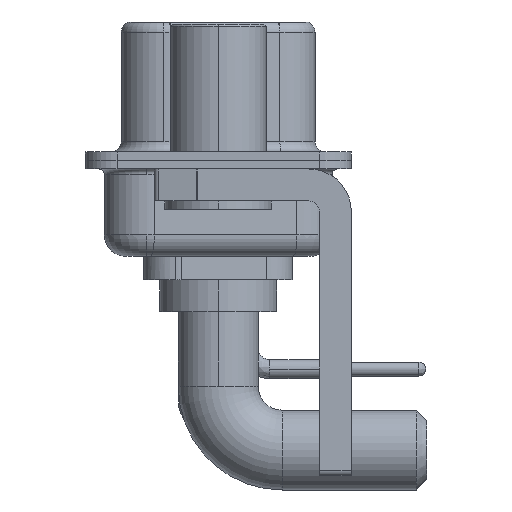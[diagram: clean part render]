
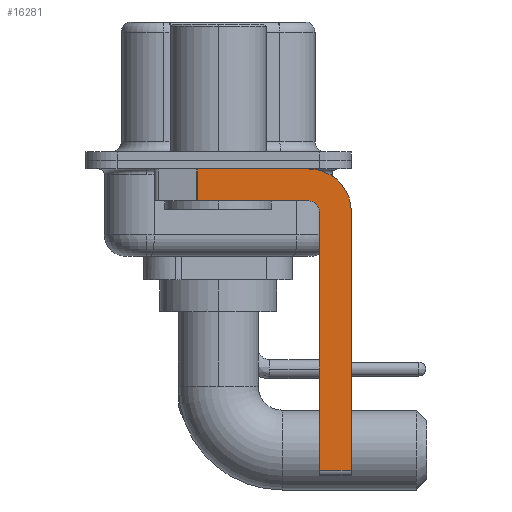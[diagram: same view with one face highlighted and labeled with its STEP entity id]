
A CAD part, left-side view. The second image highlights one B-rep face of the part: STEP entity #16281.
In plain terms, the highlighted planar face has unit normal (-1, 0, 0).
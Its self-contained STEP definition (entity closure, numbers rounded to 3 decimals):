
#114 = CARTESIAN_POINT ( 'NONE',  ( -2.9, -4.75, -14.55 ) ) ;
#766 = PLANE ( 'NONE',  #11342 ) ;
#829 = AXIS2_PLACEMENT_3D ( 'NONE', #30278, #24934, #20228 ) ;
#917 = DIRECTION ( 'NONE',  ( 0., 0., -1. ) ) ;
#1268 = VERTEX_POINT ( 'NONE', #13656 ) ;
#1734 = EDGE_CURVE ( 'NONE', #8570, #30582, #24384, .T. ) ;
#3260 = DIRECTION ( 'NONE',  ( 1., 0., 0. ) ) ;
#5506 = LINE ( 'NONE', #14772, #15397 ) ;
#5513 = EDGE_CURVE ( 'NONE', #26261, #11676, #11392, .T. ) ;
#5656 = CARTESIAN_POINT ( 'NONE',  ( -2.9, -4.75, -2.4 ) ) ;
#6050 = CARTESIAN_POINT ( 'NONE',  ( -2.9, -4.25, -2.4 ) ) ;
#6132 = EDGE_LOOP ( 'NONE', ( #12353, #15788, #12159, #10398, #16314, #27334, #27107, #17771 ) ) ;
#6307 = DIRECTION ( 'NONE',  ( 0., 0., -1. ) ) ;
#7165 = DIRECTION ( 'NONE',  ( 0., -1., 0. ) ) ;
#8091 = DIRECTION ( 'NONE',  ( 1., 0., 0. ) ) ;
#8570 = VERTEX_POINT ( 'NONE', #5656 ) ;
#8659 = CARTESIAN_POINT ( 'NONE',  ( -2.9, 0.978, -1.9 ) ) ;
#10398 = ORIENTED_EDGE ( 'NONE', *, *, #1734, .F. ) ;
#10768 = CARTESIAN_POINT ( 'NONE',  ( -2.9, 0.978, -0.4 ) ) ;
#11250 = EDGE_CURVE ( 'NONE', #11676, #1268, #25630, .T. ) ;
#11342 = AXIS2_PLACEMENT_3D ( 'NONE', #15207, #3260, #917 ) ;
#11392 = LINE ( 'NONE', #13289, #28245 ) ;
#11676 = VERTEX_POINT ( 'NONE', #26122 ) ;
#12008 = VERTEX_POINT ( 'NONE', #12074 ) ;
#12074 = CARTESIAN_POINT ( 'NONE',  ( -2.9, 0.978, -1.9 ) ) ;
#12159 = ORIENTED_EDGE ( 'NONE', *, *, #21912, .F. ) ;
#12353 = ORIENTED_EDGE ( 'NONE', *, *, #5513, .F. ) ;
#12470 = VERTEX_POINT ( 'NONE', #114 ) ;
#12634 = LINE ( 'NONE', #24431, #13814 ) ;
#13289 = CARTESIAN_POINT ( 'NONE',  ( -2.9, 3., -0.4 ) ) ;
#13373 = VERTEX_POINT ( 'NONE', #30831 ) ;
#13656 = CARTESIAN_POINT ( 'NONE',  ( -2.9, -6.25, -2.4 ) ) ;
#13814 = VECTOR ( 'NONE', #7165, 1000. ) ;
#14609 = AXIS2_PLACEMENT_3D ( 'NONE', #6050, #8091, #17840 ) ;
#14772 = CARTESIAN_POINT ( 'NONE',  ( -2.9, -4.75, -14.8 ) ) ;
#15166 = CARTESIAN_POINT ( 'NONE',  ( -2.9, -4.25, -1.9 ) ) ;
#15207 = CARTESIAN_POINT ( 'NONE',  ( -2.9, -4.25, -2.4 ) ) ;
#15327 = EDGE_CURVE ( 'NONE', #12470, #13373, #12634, .T. ) ;
#15397 = VECTOR ( 'NONE', #29210, 1000. ) ;
#15788 = ORIENTED_EDGE ( 'NONE', *, *, #19373, .T. ) ;
#16205 = VECTOR ( 'NONE', #29453, 1000. ) ;
#16281 = ADVANCED_FACE ( 'NONE', ( #22269 ), #766, .F. ) ;
#16314 = ORIENTED_EDGE ( 'NONE', *, *, #18359, .F. ) ;
#17002 = CARTESIAN_POINT ( 'NONE',  ( -2.9, -6.25, -2.4 ) ) ;
#17771 = ORIENTED_EDGE ( 'NONE', *, *, #11250, .F. ) ;
#17840 = DIRECTION ( 'NONE',  ( 0., 0., -1. ) ) ;
#18359 = EDGE_CURVE ( 'NONE', #12470, #8570, #5506, .T. ) ;
#18731 = LINE ( 'NONE', #17002, #25343 ) ;
#19373 = EDGE_CURVE ( 'NONE', #26261, #12008, #27505, .T. ) ;
#20228 = DIRECTION ( 'NONE',  ( 0., 0., 1. ) ) ;
#20984 = DIRECTION ( 'NONE',  ( 0., -1., 0. ) ) ;
#21912 = EDGE_CURVE ( 'NONE', #30582, #12008, #24580, .T. ) ;
#22269 = FACE_OUTER_BOUND ( 'NONE', #6132, .T. ) ;
#23938 = EDGE_CURVE ( 'NONE', #1268, #13373, #18731, .T. ) ;
#24297 = CARTESIAN_POINT ( 'NONE',  ( -2.9, -4.25, -1.9 ) ) ;
#24384 = CIRCLE ( 'NONE', #829, 0.5 ) ;
#24431 = CARTESIAN_POINT ( 'NONE',  ( -2.9, -4.25, -14.55 ) ) ;
#24468 = VECTOR ( 'NONE', #6307, 1000. ) ;
#24580 = LINE ( 'NONE', #15166, #16205 ) ;
#24934 = DIRECTION ( 'NONE',  ( -1., 0., 0. ) ) ;
#25343 = VECTOR ( 'NONE', #26259, 1000. ) ;
#25630 = CIRCLE ( 'NONE', #14609, 2. ) ;
#26122 = CARTESIAN_POINT ( 'NONE',  ( -2.9, -4.25, -0.4 ) ) ;
#26259 = DIRECTION ( 'NONE',  ( 0., 0., -1. ) ) ;
#26261 = VERTEX_POINT ( 'NONE', #10768 ) ;
#27107 = ORIENTED_EDGE ( 'NONE', *, *, #23938, .F. ) ;
#27334 = ORIENTED_EDGE ( 'NONE', *, *, #15327, .T. ) ;
#27505 = LINE ( 'NONE', #8659, #24468 ) ;
#28245 = VECTOR ( 'NONE', #20984, 1000. ) ;
#29210 = DIRECTION ( 'NONE',  ( 0., 0., 1. ) ) ;
#29453 = DIRECTION ( 'NONE',  ( 0., 1., 0. ) ) ;
#30278 = CARTESIAN_POINT ( 'NONE',  ( -2.9, -4.25, -2.4 ) ) ;
#30582 = VERTEX_POINT ( 'NONE', #24297 ) ;
#30831 = CARTESIAN_POINT ( 'NONE',  ( -2.9, -6.25, -14.55 ) ) ;
